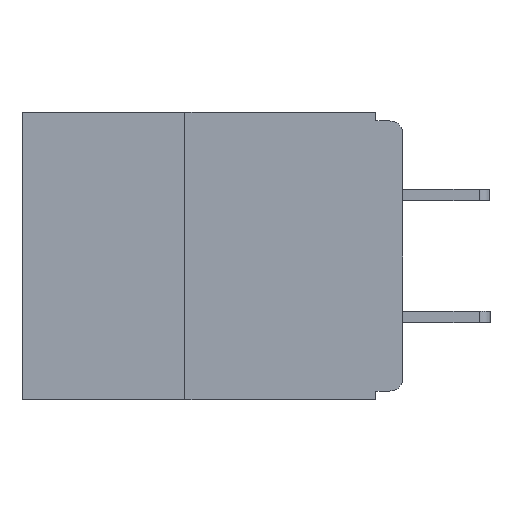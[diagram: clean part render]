
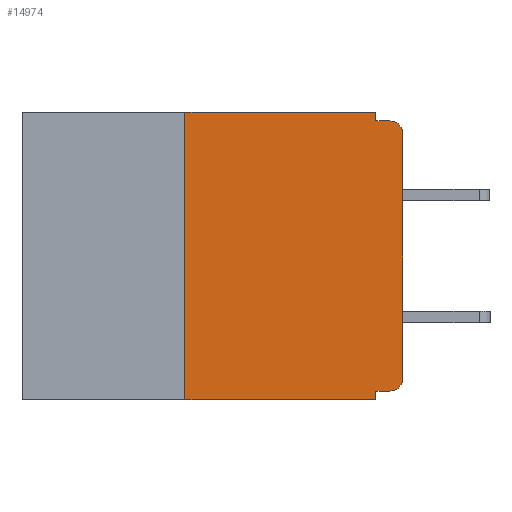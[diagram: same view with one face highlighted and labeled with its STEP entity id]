
A CAD part, left-side view. The second image highlights one B-rep face of the part: STEP entity #14974.
In plain terms, the highlighted planar face has unit normal (-1, 0, 0).
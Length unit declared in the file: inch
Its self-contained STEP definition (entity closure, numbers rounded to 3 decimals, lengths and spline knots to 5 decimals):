
#117 = CARTESIAN_POINT ( 'NONE',  ( 0., 0.25, -0.33 ) ) ;
#465 = EDGE_LOOP ( 'NONE', ( #5679, #4691, #10748, #10090, #5477, #11736, #8833, #7036, #2355, #14138 ) ) ;
#488 = AXIS2_PLACEMENT_3D ( 'NONE', #2463, #2387, #4548 ) ;
#1021 = CARTESIAN_POINT ( 'NONE',  ( 0., 0.031, 0. ) ) ;
#1031 = VECTOR ( 'NONE', #19903, 39.37008 ) ;
#1235 = LINE ( 'NONE', #12116, #5516 ) ;
#1777 = CARTESIAN_POINT ( 'NONE',  ( 0., 0.015, -0.025 ) ) ;
#1957 = CIRCLE ( 'NONE', #488, 0.015 ) ;
#2355 = ORIENTED_EDGE ( 'NONE', *, *, #12420, .F. ) ;
#2387 = DIRECTION ( 'NONE',  ( -1., 0., 0. ) ) ;
#2463 = CARTESIAN_POINT ( 'NONE',  ( 0., 0.015, -0.305 ) ) ;
#3352 = CARTESIAN_POINT ( 'NONE',  ( 0., 0.031, -0.32 ) ) ;
#3358 = DIRECTION ( 'NONE',  ( 0., 0., -1. ) ) ;
#3422 = DIRECTION ( 'NONE',  ( 0., 0., -1. ) ) ;
#3664 = EDGE_CURVE ( 'NONE', #18651, #20380, #14463, .T. ) ;
#3736 = LINE ( 'NONE', #5826, #15600 ) ;
#4101 = DIRECTION ( 'NONE',  ( 0., -1., 0. ) ) ;
#4190 = EDGE_CURVE ( 'NONE', #10261, #20380, #5326, .T. ) ;
#4308 = VERTEX_POINT ( 'NONE', #1021 ) ;
#4548 = DIRECTION ( 'NONE',  ( 0., 0., -1. ) ) ;
#4576 = VECTOR ( 'NONE', #15975, 39.37008 ) ;
#4597 = CARTESIAN_POINT ( 'NONE',  ( 0., 0., -0.025 ) ) ;
#4691 = ORIENTED_EDGE ( 'NONE', *, *, #20471, .T. ) ;
#5225 = CARTESIAN_POINT ( 'NONE',  ( 0., 0.25, 0. ) ) ;
#5326 = LINE ( 'NONE', #12020, #1031 ) ;
#5367 = VECTOR ( 'NONE', #3358, 39.37008 ) ;
#5477 = ORIENTED_EDGE ( 'NONE', *, *, #15966, .F. ) ;
#5516 = VECTOR ( 'NONE', #4101, 39.37008 ) ;
#5679 = ORIENTED_EDGE ( 'NONE', *, *, #10776, .T. ) ;
#5826 = CARTESIAN_POINT ( 'NONE',  ( 0., 0., -0.32 ) ) ;
#5855 = EDGE_CURVE ( 'NONE', #12530, #9472, #1957, .T. ) ;
#6256 = EDGE_CURVE ( 'NONE', #14152, #18650, #7256, .T. ) ;
#7036 = ORIENTED_EDGE ( 'NONE', *, *, #3664, .F. ) ;
#7256 = LINE ( 'NONE', #19056, #7757 ) ;
#7326 = DIRECTION ( 'NONE',  ( 0., 0., -1. ) ) ;
#7757 = VECTOR ( 'NONE', #19014, 39.37008 ) ;
#8407 = CARTESIAN_POINT ( 'NONE',  ( 0., 0.031, -0.33 ) ) ;
#8833 = ORIENTED_EDGE ( 'NONE', *, *, #4190, .T. ) ;
#9472 = VERTEX_POINT ( 'NONE', #18659 ) ;
#9679 = EDGE_CURVE ( 'NONE', #4308, #14152, #10204, .T. ) ;
#9682 = CIRCLE ( 'NONE', #15212, 0.015 ) ;
#9836 = EDGE_CURVE ( 'NONE', #10261, #18778, #18858, .T. ) ;
#10090 = ORIENTED_EDGE ( 'NONE', *, *, #9679, .F. ) ;
#10186 = VECTOR ( 'NONE', #11547, 39.37008 ) ;
#10204 = LINE ( 'NONE', #19314, #5367 ) ;
#10261 = VERTEX_POINT ( 'NONE', #117 ) ;
#10431 = VECTOR ( 'NONE', #13515, 39.37008 ) ;
#10748 = ORIENTED_EDGE ( 'NONE', *, *, #6256, .F. ) ;
#10776 = EDGE_CURVE ( 'NONE', #9472, #19155, #17356, .T. ) ;
#11547 = DIRECTION ( 'NONE',  ( 0., 0., -1. ) ) ;
#11736 = ORIENTED_EDGE ( 'NONE', *, *, #9836, .F. ) ;
#12020 = CARTESIAN_POINT ( 'NONE',  ( 0., 0.437, -0.33 ) ) ;
#12116 = CARTESIAN_POINT ( 'NONE',  ( 0., 0.437, 0. ) ) ;
#12420 = EDGE_CURVE ( 'NONE', #12530, #18651, #3736, .T. ) ;
#12530 = VERTEX_POINT ( 'NONE', #16948 ) ;
#12796 = CARTESIAN_POINT ( 'NONE',  ( 0., 0.031, -0.33 ) ) ;
#13002 = CARTESIAN_POINT ( 'NONE',  ( 0., 0.015, -0.01 ) ) ;
#13080 = DIRECTION ( 'NONE',  ( -1., 0., 0. ) ) ;
#13515 = DIRECTION ( 'NONE',  ( 0., 0., 1. ) ) ;
#13757 = PLANE ( 'NONE',  #16802 ) ;
#14138 = ORIENTED_EDGE ( 'NONE', *, *, #5855, .T. ) ;
#14152 = VERTEX_POINT ( 'NONE', #16816 ) ;
#14388 = CARTESIAN_POINT ( 'NONE',  ( 0., 0., 0. ) ) ;
#14463 = LINE ( 'NONE', #8407, #10186 ) ;
#14974 = ADVANCED_FACE ( 'NONE', ( #19346 ), #13757, .F. ) ;
#15067 = CARTESIAN_POINT ( 'NONE',  ( 0., 0.25, -0.33 ) ) ;
#15212 = AXIS2_PLACEMENT_3D ( 'NONE', #1777, #13080, #3422 ) ;
#15381 = CARTESIAN_POINT ( 'NONE',  ( 0., 0.437, 0. ) ) ;
#15513 = DIRECTION ( 'NONE',  ( 0., 1., 0. ) ) ;
#15600 = VECTOR ( 'NONE', #15513, 39.37008 ) ;
#15966 = EDGE_CURVE ( 'NONE', #18778, #4308, #1235, .T. ) ;
#15975 = DIRECTION ( 'NONE',  ( 0., 0., 1. ) ) ;
#16802 = AXIS2_PLACEMENT_3D ( 'NONE', #15381, #16928, #7326 ) ;
#16816 = CARTESIAN_POINT ( 'NONE',  ( 0., 0.031, -0.01 ) ) ;
#16928 = DIRECTION ( 'NONE',  ( 1., 0., 0. ) ) ;
#16948 = CARTESIAN_POINT ( 'NONE',  ( 0., 0.015, -0.32 ) ) ;
#17356 = LINE ( 'NONE', #14388, #4576 ) ;
#18650 = VERTEX_POINT ( 'NONE', #13002 ) ;
#18651 = VERTEX_POINT ( 'NONE', #3352 ) ;
#18659 = CARTESIAN_POINT ( 'NONE',  ( 0., 0., -0.305 ) ) ;
#18778 = VERTEX_POINT ( 'NONE', #5225 ) ;
#18858 = LINE ( 'NONE', #15067, #10431 ) ;
#19014 = DIRECTION ( 'NONE',  ( 0., -1., 0. ) ) ;
#19056 = CARTESIAN_POINT ( 'NONE',  ( 0., 0., -0.01 ) ) ;
#19155 = VERTEX_POINT ( 'NONE', #4597 ) ;
#19314 = CARTESIAN_POINT ( 'NONE',  ( 0., 0.031, 0. ) ) ;
#19346 = FACE_OUTER_BOUND ( 'NONE', #465, .T. ) ;
#19903 = DIRECTION ( 'NONE',  ( 0., -1., 0. ) ) ;
#20380 = VERTEX_POINT ( 'NONE', #12796 ) ;
#20471 = EDGE_CURVE ( 'NONE', #19155, #18650, #9682, .T. ) ;
